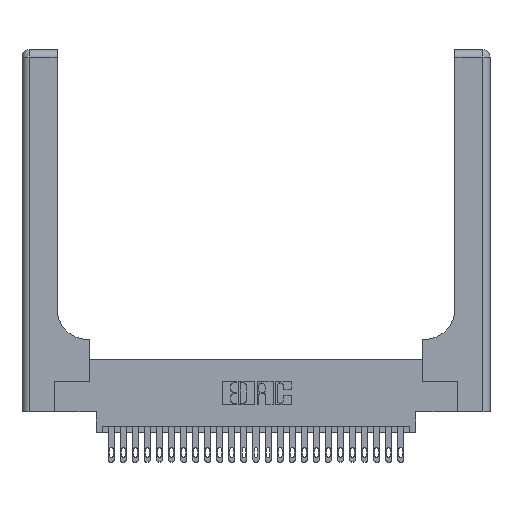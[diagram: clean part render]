
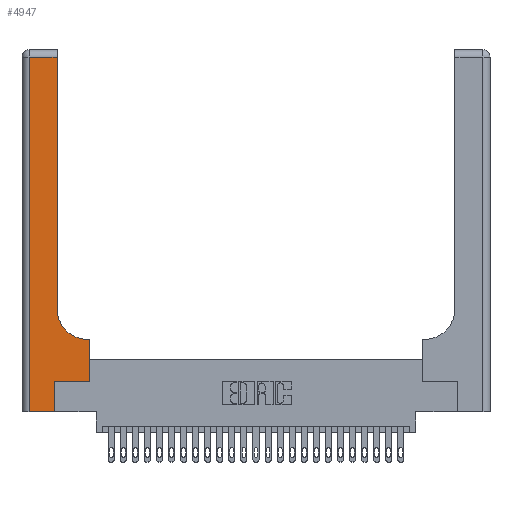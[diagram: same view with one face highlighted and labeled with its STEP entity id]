
A CAD part, top view. The second image highlights one B-rep face of the part: STEP entity #4947.
In plain terms, the highlighted planar face has unit normal (0, 0, 1).
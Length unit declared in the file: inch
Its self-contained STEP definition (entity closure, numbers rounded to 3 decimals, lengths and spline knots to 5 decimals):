
#953 = CARTESIAN_POINT ( 'NONE',  ( 0.5585, 0.6, 0.37 ) ) ;
#2017 = VECTOR ( 'NONE', #25911, 39.37008 ) ;
#2899 = ORIENTED_EDGE ( 'NONE', *, *, #9532, .T. ) ;
#2943 = AXIS2_PLACEMENT_3D ( 'NONE', #24570, #26567, #9797 ) ;
#3311 = LINE ( 'NONE', #21286, #5946 ) ;
#3590 = ORIENTED_EDGE ( 'NONE', *, *, #12801, .T. ) ;
#3703 = LINE ( 'NONE', #23551, #2017 ) ;
#4746 = ORIENTED_EDGE ( 'NONE', *, *, #8648, .T. ) ;
#4947 = ADVANCED_FACE ( 'NONE', ( #8148 ), #24387, .F. ) ;
#5256 = EDGE_CURVE ( 'NONE', #8409, #24536, #24150, .T. ) ;
#5946 = VECTOR ( 'NONE', #15111, 39.37008 ) ;
#6441 = CARTESIAN_POINT ( 'NONE',  ( 0.2915, 0.6, 0.37 ) ) ;
#6817 = CARTESIAN_POINT ( 'NONE',  ( 0.5585, 0.25, 0.37 ) ) ;
#6935 = CARTESIAN_POINT ( 'NONE',  ( 0.2915, 3., 0.37 ) ) ;
#7021 = DIRECTION ( 'NONE',  ( 0., 1., 0. ) ) ;
#7767 = VECTOR ( 'NONE', #21236, 39.37008 ) ;
#8148 = FACE_OUTER_BOUND ( 'NONE', #18176, .T. ) ;
#8409 = VERTEX_POINT ( 'NONE', #25083 ) ;
#8648 = EDGE_CURVE ( 'NONE', #25707, #12468, #20055, .T. ) ;
#9532 = EDGE_CURVE ( 'NONE', #24343, #25707, #15394, .T. ) ;
#9731 = ORIENTED_EDGE ( 'NONE', *, *, #5256, .T. ) ;
#9797 = DIRECTION ( 'NONE',  ( -1., 0., 0. ) ) ;
#10155 = DIRECTION ( 'NONE',  ( 1., 0., 0. ) ) ;
#10639 = DIRECTION ( 'NONE',  ( -1., 0., 0. ) ) ;
#10907 = LINE ( 'NONE', #13249, #20108 ) ;
#11344 = ORIENTED_EDGE ( 'NONE', *, *, #26058, .T. ) ;
#12468 = VERTEX_POINT ( 'NONE', #14151 ) ;
#12748 = VERTEX_POINT ( 'NONE', #16703 ) ;
#12801 = EDGE_CURVE ( 'NONE', #20047, #21841, #22592, .T. ) ;
#13249 = CARTESIAN_POINT ( 'NONE',  ( 0.269, 0.25, 0.37 ) ) ;
#14151 = CARTESIAN_POINT ( 'NONE',  ( 0.2915, 2.94, 0.37 ) ) ;
#14425 = CARTESIAN_POINT ( 'NONE',  ( 0., 0., 0.37 ) ) ;
#14430 = VECTOR ( 'NONE', #7021, 39.37008 ) ;
#15111 = DIRECTION ( 'NONE',  ( 0., 1., 0. ) ) ;
#15394 = CIRCLE ( 'NONE', #17737, 0.25 ) ;
#15469 = DIRECTION ( 'NONE',  ( 1., 0., 0. ) ) ;
#16146 = EDGE_CURVE ( 'NONE', #21841, #24343, #23454, .T. ) ;
#16339 = VECTOR ( 'NONE', #25429, 39.37008 ) ;
#16703 = CARTESIAN_POINT ( 'NONE',  ( 0.269, 0., 0.37 ) ) ;
#16801 = CARTESIAN_POINT ( 'NONE',  ( 0.06, 3., 0.37 ) ) ;
#16876 = EDGE_CURVE ( 'NONE', #20100, #20047, #10907, .T. ) ;
#17114 = VECTOR ( 'NONE', #10155, 39.37008 ) ;
#17290 = CARTESIAN_POINT ( 'NONE',  ( 0.5415, 0.85, 0.37 ) ) ;
#17737 = AXIS2_PLACEMENT_3D ( 'NONE', #17290, #25948, #15469 ) ;
#18176 = EDGE_LOOP ( 'NONE', ( #4746, #21910, #9731, #11344, #22697, #20270, #3590, #19041, #2899 ) ) ;
#18202 = CARTESIAN_POINT ( 'NONE',  ( 0.5415, 0.6, 0.37 ) ) ;
#19041 = ORIENTED_EDGE ( 'NONE', *, *, #16146, .T. ) ;
#19704 = DIRECTION ( 'NONE',  ( 1., 0., 0. ) ) ;
#20047 = VERTEX_POINT ( 'NONE', #6817 ) ;
#20055 = LINE ( 'NONE', #6935, #14430 ) ;
#20100 = VERTEX_POINT ( 'NONE', #23606 ) ;
#20108 = VECTOR ( 'NONE', #19704, 39.37008 ) ;
#20270 = ORIENTED_EDGE ( 'NONE', *, *, #16876, .T. ) ;
#21236 = DIRECTION ( 'NONE',  ( 0., -1., 0. ) ) ;
#21286 = CARTESIAN_POINT ( 'NONE',  ( 0.269, 0., 0.37 ) ) ;
#21841 = VERTEX_POINT ( 'NONE', #953 ) ;
#21910 = ORIENTED_EDGE ( 'NONE', *, *, #26290, .T. ) ;
#22592 = LINE ( 'NONE', #25704, #16339 ) ;
#22697 = ORIENTED_EDGE ( 'NONE', *, *, #27041, .T. ) ;
#23214 = CARTESIAN_POINT ( 'NONE',  ( 0.2915, 0.85, 0.37 ) ) ;
#23454 = LINE ( 'NONE', #6441, #26059 ) ;
#23551 = CARTESIAN_POINT ( 'NONE',  ( 0., 2.94, 0.37 ) ) ;
#23606 = CARTESIAN_POINT ( 'NONE',  ( 0.269, 0.25, 0.37 ) ) ;
#24061 = LINE ( 'NONE', #14425, #17114 ) ;
#24150 = LINE ( 'NONE', #16801, #7767 ) ;
#24343 = VERTEX_POINT ( 'NONE', #18202 ) ;
#24387 = PLANE ( 'NONE',  #2943 ) ;
#24536 = VERTEX_POINT ( 'NONE', #25372 ) ;
#24570 = CARTESIAN_POINT ( 'NONE',  ( 0., 3., 0.37 ) ) ;
#25083 = CARTESIAN_POINT ( 'NONE',  ( 0.06, 2.94, 0.37 ) ) ;
#25372 = CARTESIAN_POINT ( 'NONE',  ( 0.06, 0., 0.37 ) ) ;
#25429 = DIRECTION ( 'NONE',  ( 0., 1., 0. ) ) ;
#25704 = CARTESIAN_POINT ( 'NONE',  ( 0.5585, 0.25, 0.37 ) ) ;
#25707 = VERTEX_POINT ( 'NONE', #23214 ) ;
#25911 = DIRECTION ( 'NONE',  ( -1., 0., 0. ) ) ;
#25948 = DIRECTION ( 'NONE',  ( 0., 0., -1. ) ) ;
#26058 = EDGE_CURVE ( 'NONE', #24536, #12748, #24061, .T. ) ;
#26059 = VECTOR ( 'NONE', #10639, 39.37008 ) ;
#26290 = EDGE_CURVE ( 'NONE', #12468, #8409, #3703, .T. ) ;
#26567 = DIRECTION ( 'NONE',  ( 0., 0., -1. ) ) ;
#27041 = EDGE_CURVE ( 'NONE', #12748, #20100, #3311, .T. ) ;
